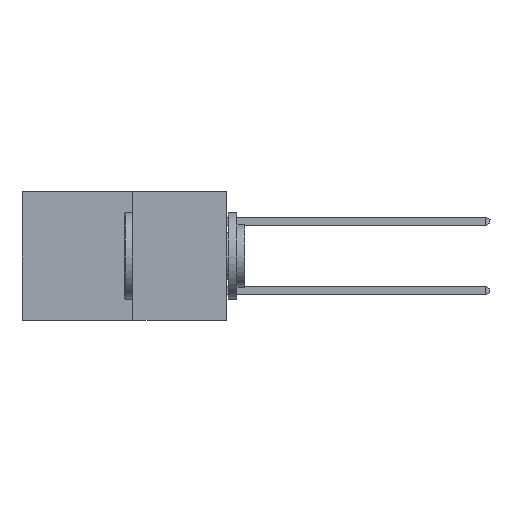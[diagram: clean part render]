
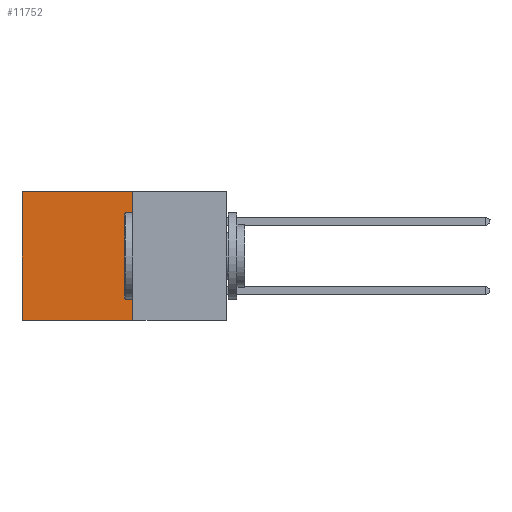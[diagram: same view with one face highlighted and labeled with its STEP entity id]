
A CAD part, left-side view. The second image highlights one B-rep face of the part: STEP entity #11752.
In plain terms, the highlighted planar face has unit normal (-1, 0, 0).
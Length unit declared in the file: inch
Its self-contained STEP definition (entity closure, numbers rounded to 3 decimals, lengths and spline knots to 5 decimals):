
#101 = ORIENTED_EDGE ( 'NONE', *, *, #23569, .T. ) ;
#3179 = PLANE ( 'NONE',  #12869 ) ;
#4877 = LINE ( 'NONE', #29016, #30148 ) ;
#5010 = LINE ( 'NONE', #13669, #26035 ) ;
#6963 = DIRECTION ( 'NONE',  ( 0., 0., -1. ) ) ;
#7354 = CARTESIAN_POINT ( 'NONE',  ( 0.277, 0.27, 0. ) ) ;
#8212 = VERTEX_POINT ( 'NONE', #9345 ) ;
#8275 = CARTESIAN_POINT ( 'NONE',  ( 0.277, 0.27, -0.37 ) ) ;
#8363 = CARTESIAN_POINT ( 'NONE',  ( 0.277, 0.59, 0. ) ) ;
#9345 = CARTESIAN_POINT ( 'NONE',  ( 0.277, 0.27, -0.37 ) ) ;
#10756 = ORIENTED_EDGE ( 'NONE', *, *, #22518, .F. ) ;
#10831 = DIRECTION ( 'NONE',  ( 0., 0., -1. ) ) ;
#11752 = ADVANCED_FACE ( 'NONE', ( #22177 ), #3179, .F. ) ;
#11973 = VERTEX_POINT ( 'NONE', #21757 ) ;
#12573 = EDGE_CURVE ( 'NONE', #8212, #11973, #5010, .T. ) ;
#12869 = AXIS2_PLACEMENT_3D ( 'NONE', #8275, #26020, #10831 ) ;
#13669 = CARTESIAN_POINT ( 'NONE',  ( 0.277, 0.27, -0.37 ) ) ;
#13898 = VERTEX_POINT ( 'NONE', #8363 ) ;
#14054 = LINE ( 'NONE', #27117, #27525 ) ;
#17063 = LINE ( 'NONE', #7354, #30402 ) ;
#17111 = EDGE_CURVE ( 'NONE', #17738, #13898, #17063, .T. ) ;
#17738 = VERTEX_POINT ( 'NONE', #29740 ) ;
#19049 = DIRECTION ( 'NONE',  ( 0., 0., -1. ) ) ;
#21757 = CARTESIAN_POINT ( 'NONE',  ( 0.277, 0.59, -0.37 ) ) ;
#22177 = FACE_OUTER_BOUND ( 'NONE', #26257, .T. ) ;
#22518 = EDGE_CURVE ( 'NONE', #17738, #8212, #14054, .T. ) ;
#23569 = EDGE_CURVE ( 'NONE', #13898, #11973, #4877, .T. ) ;
#26020 = DIRECTION ( 'NONE',  ( 1., 0., 0. ) ) ;
#26035 = VECTOR ( 'NONE', #31260, 39.37008 ) ;
#26257 = EDGE_LOOP ( 'NONE', ( #101, #29331, #10756, #27320 ) ) ;
#27117 = CARTESIAN_POINT ( 'NONE',  ( 0.277, 0.27, -0.37 ) ) ;
#27320 = ORIENTED_EDGE ( 'NONE', *, *, #17111, .T. ) ;
#27525 = VECTOR ( 'NONE', #6963, 39.37008 ) ;
#27628 = DIRECTION ( 'NONE',  ( 0., 1., 0. ) ) ;
#29016 = CARTESIAN_POINT ( 'NONE',  ( 0.277, 0.59, -0.37 ) ) ;
#29331 = ORIENTED_EDGE ( 'NONE', *, *, #12573, .F. ) ;
#29740 = CARTESIAN_POINT ( 'NONE',  ( 0.277, 0.27, 0. ) ) ;
#30148 = VECTOR ( 'NONE', #19049, 39.37008 ) ;
#30402 = VECTOR ( 'NONE', #27628, 39.37008 ) ;
#31260 = DIRECTION ( 'NONE',  ( 0., 1., 0. ) ) ;
